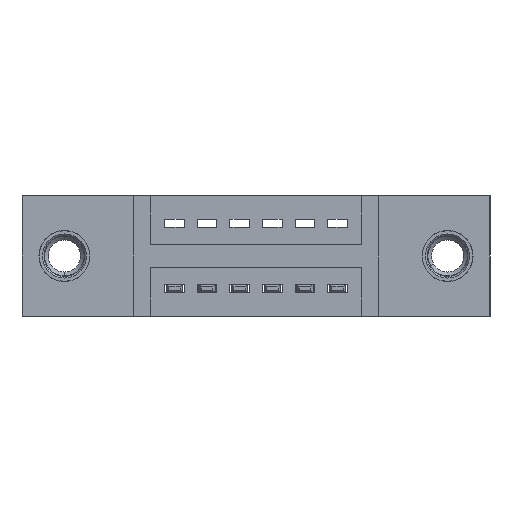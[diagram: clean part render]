
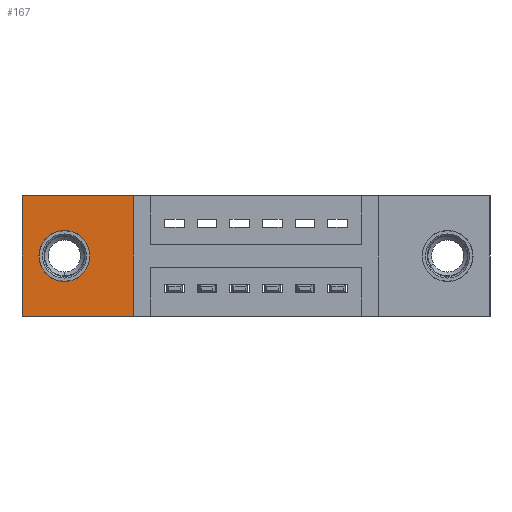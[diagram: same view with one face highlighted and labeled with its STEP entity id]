
A CAD part, front view. The second image highlights one B-rep face of the part: STEP entity #167.
In plain terms, the highlighted planar face has unit normal (0, -1, 0).
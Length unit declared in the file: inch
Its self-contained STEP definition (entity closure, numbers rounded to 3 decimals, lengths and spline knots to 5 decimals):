
#120 = CARTESIAN_POINT ( 'NONE',  ( 0.3425, 0.11, 0. ) ) ;
#167 = ADVANCED_FACE ( 'NONE', ( #302, #3721 ), #254, .T. ) ;
#254 = PLANE ( 'NONE',  #10117 ) ;
#298 = LINE ( 'NONE', #7363, #3825 ) ;
#302 = FACE_BOUND ( 'NONE', #9803, .T. ) ;
#1028 = CARTESIAN_POINT ( 'NONE',  ( 0.13, 0.11, -0.107 ) ) ;
#1062 = DIRECTION ( 'NONE',  ( 0., 0., -1. ) ) ;
#1068 = DIRECTION ( 'NONE',  ( 0., 0., -1. ) ) ;
#1075 = CARTESIAN_POINT ( 'NONE',  ( 0., 0.11, 0. ) ) ;
#1217 = VERTEX_POINT ( 'NONE', #6356 ) ;
#1322 = DIRECTION ( 'NONE',  ( 1., 0., 0. ) ) ;
#1779 = ORIENTED_EDGE ( 'NONE', *, *, #6220, .F. ) ;
#1883 = CARTESIAN_POINT ( 'NONE',  ( 0., 0.11, -0.37 ) ) ;
#2313 = DIRECTION ( 'NONE',  ( 0., -1., 0. ) ) ;
#3015 = DIRECTION ( 'NONE',  ( -1., 0., 0. ) ) ;
#3110 = EDGE_CURVE ( 'NONE', #3906, #7269, #9198, .T. ) ;
#3163 = DIRECTION ( 'NONE',  ( 0., 0., -1. ) ) ;
#3303 = LINE ( 'NONE', #1075, #9543 ) ;
#3702 = LINE ( 'NONE', #8652, #8920 ) ;
#3721 = FACE_OUTER_BOUND ( 'NONE', #7860, .T. ) ;
#3825 = VECTOR ( 'NONE', #9034, 39.37008 ) ;
#3853 = CARTESIAN_POINT ( 'NONE',  ( 0., 0.11, 0. ) ) ;
#3906 = VERTEX_POINT ( 'NONE', #1028 ) ;
#3940 = CARTESIAN_POINT ( 'NONE',  ( 0.13, 0.11, -0.185 ) ) ;
#4172 = EDGE_CURVE ( 'NONE', #1217, #7990, #3303, .T. ) ;
#4247 = VERTEX_POINT ( 'NONE', #4988 ) ;
#4391 = ORIENTED_EDGE ( 'NONE', *, *, #10360, .T. ) ;
#4802 = EDGE_CURVE ( 'NONE', #7469, #1217, #7898, .T. ) ;
#4988 = CARTESIAN_POINT ( 'NONE',  ( 0.3425, 0.11, -0.37 ) ) ;
#5347 = CARTESIAN_POINT ( 'NONE',  ( 0.13, 0.11, -0.263 ) ) ;
#5995 = DIRECTION ( 'NONE',  ( 0., -1., 0. ) ) ;
#6008 = DIRECTION ( 'NONE',  ( 0., 0., -1. ) ) ;
#6193 = CIRCLE ( 'NONE', #10371, 0.078 ) ;
#6220 = EDGE_CURVE ( 'NONE', #7269, #3906, #6193, .T. ) ;
#6235 = ORIENTED_EDGE ( 'NONE', *, *, #3110, .F. ) ;
#6252 = ORIENTED_EDGE ( 'NONE', *, *, #10460, .T. ) ;
#6356 = CARTESIAN_POINT ( 'NONE',  ( 0., 0.11, 0. ) ) ;
#6581 = ORIENTED_EDGE ( 'NONE', *, *, #4172, .T. ) ;
#7269 = VERTEX_POINT ( 'NONE', #5347 ) ;
#7363 = CARTESIAN_POINT ( 'NONE',  ( 0.3425, 0.11, 0. ) ) ;
#7469 = VERTEX_POINT ( 'NONE', #120 ) ;
#7549 = CARTESIAN_POINT ( 'NONE',  ( 0., 0.11, -0.37 ) ) ;
#7860 = EDGE_LOOP ( 'NONE', ( #6581, #6252, #4391, #9836 ) ) ;
#7898 = LINE ( 'NONE', #3853, #10292 ) ;
#7990 = VERTEX_POINT ( 'NONE', #7549 ) ;
#8248 = CARTESIAN_POINT ( 'NONE',  ( 0.13, 0.11, -0.185 ) ) ;
#8280 = DIRECTION ( 'NONE',  ( 0., -1., 0. ) ) ;
#8652 = CARTESIAN_POINT ( 'NONE',  ( 0., 0.11, -0.37 ) ) ;
#8920 = VECTOR ( 'NONE', #1322, 39.37008 ) ;
#8943 = AXIS2_PLACEMENT_3D ( 'NONE', #3940, #2313, #3163 ) ;
#9034 = DIRECTION ( 'NONE',  ( 0., 0., 1. ) ) ;
#9198 = CIRCLE ( 'NONE', #8943, 0.078 ) ;
#9543 = VECTOR ( 'NONE', #6008, 39.37008 ) ;
#9803 = EDGE_LOOP ( 'NONE', ( #6235, #1779 ) ) ;
#9836 = ORIENTED_EDGE ( 'NONE', *, *, #4802, .T. ) ;
#10117 = AXIS2_PLACEMENT_3D ( 'NONE', #1883, #5995, #1062 ) ;
#10292 = VECTOR ( 'NONE', #3015, 39.37008 ) ;
#10360 = EDGE_CURVE ( 'NONE', #4247, #7469, #298, .T. ) ;
#10371 = AXIS2_PLACEMENT_3D ( 'NONE', #8248, #8280, #1068 ) ;
#10460 = EDGE_CURVE ( 'NONE', #7990, #4247, #3702, .T. ) ;
